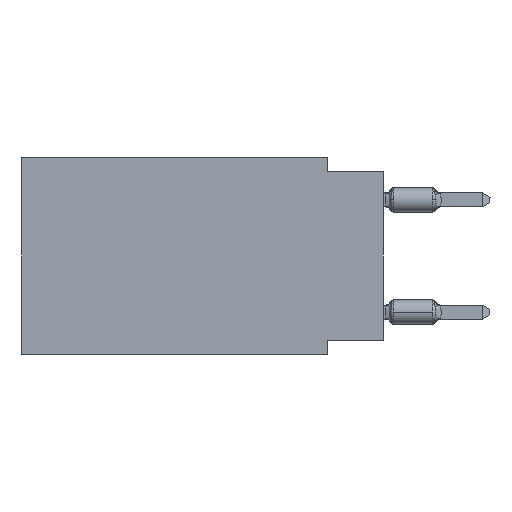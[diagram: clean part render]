
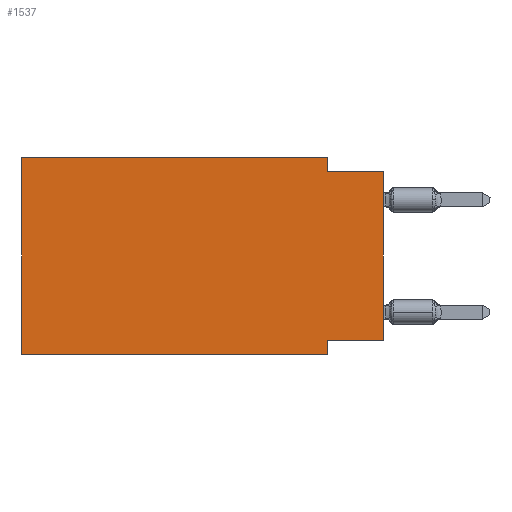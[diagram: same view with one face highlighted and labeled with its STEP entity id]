
A CAD part, left-side view. The second image highlights one B-rep face of the part: STEP entity #1537.
In plain terms, the highlighted planar face has unit normal (-1, 0, 0).
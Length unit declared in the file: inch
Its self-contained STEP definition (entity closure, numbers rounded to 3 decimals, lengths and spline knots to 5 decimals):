
#310 = VERTEX_POINT ( 'NONE', #21099 ) ;
#391 = EDGE_CURVE ( 'NONE', #17264, #3474, #10480, .T. ) ;
#471 = LINE ( 'NONE', #23432, #18059 ) ;
#589 = DIRECTION ( 'NONE',  ( 0., 0., -1. ) ) ;
#600 = VERTEX_POINT ( 'NONE', #11206 ) ;
#937 = CARTESIAN_POINT ( 'NONE',  ( 0., 0.1, -0.35 ) ) ;
#1000 = DIRECTION ( 'NONE',  ( 0., 0., 1. ) ) ;
#1537 = ADVANCED_FACE ( 'NONE', ( #15249 ), #3746, .F. ) ;
#1828 = EDGE_CURVE ( 'NONE', #600, #13780, #6998, .T. ) ;
#2610 = CARTESIAN_POINT ( 'NONE',  ( 0., 0.1, -0.35 ) ) ;
#2752 = LINE ( 'NONE', #18110, #24153 ) ;
#3033 = VECTOR ( 'NONE', #6122, 39.37008 ) ;
#3474 = VERTEX_POINT ( 'NONE', #937 ) ;
#3730 = ORIENTED_EDGE ( 'NONE', *, *, #391, .F. ) ;
#3746 = PLANE ( 'NONE',  #22382 ) ;
#3873 = DIRECTION ( 'NONE',  ( 0., 0., -1. ) ) ;
#4231 = LINE ( 'NONE', #15497, #3033 ) ;
#4282 = EDGE_CURVE ( 'NONE', #310, #13780, #10447, .T. ) ;
#5043 = DIRECTION ( 'NONE',  ( 0., -1., 0. ) ) ;
#6122 = DIRECTION ( 'NONE',  ( 0., 1., 0. ) ) ;
#6454 = CARTESIAN_POINT ( 'NONE',  ( 0., 0., -0.025 ) ) ;
#6998 = LINE ( 'NONE', #14608, #18767 ) ;
#9003 = VECTOR ( 'NONE', #19560, 39.37008 ) ;
#9133 = EDGE_CURVE ( 'NONE', #23872, #18545, #9851, .T. ) ;
#9687 = ORIENTED_EDGE ( 'NONE', *, *, #23823, .F. ) ;
#9851 = LINE ( 'NONE', #15473, #15080 ) ;
#10447 = LINE ( 'NONE', #6454, #9003 ) ;
#10480 = LINE ( 'NONE', #2610, #23742 ) ;
#11206 = CARTESIAN_POINT ( 'NONE',  ( 0., 0., -0.325 ) ) ;
#11257 = CARTESIAN_POINT ( 'NONE',  ( 0., 0.645, 0. ) ) ;
#11541 = ORIENTED_EDGE ( 'NONE', *, *, #4282, .F. ) ;
#11557 = ORIENTED_EDGE ( 'NONE', *, *, #1828, .T. ) ;
#12058 = VECTOR ( 'NONE', #5043, 39.37008 ) ;
#12615 = CARTESIAN_POINT ( 'NONE',  ( 0., 0.645, 0. ) ) ;
#12748 = EDGE_CURVE ( 'NONE', #18545, #310, #471, .T. ) ;
#13166 = CARTESIAN_POINT ( 'NONE',  ( 0., 0.1, 0. ) ) ;
#13590 = DIRECTION ( 'NONE',  ( 0., -1., 0. ) ) ;
#13748 = CARTESIAN_POINT ( 'NONE',  ( 0., 0.645, -0.35 ) ) ;
#13780 = VERTEX_POINT ( 'NONE', #19332 ) ;
#13970 = DIRECTION ( 'NONE',  ( 0., 0., -1. ) ) ;
#14608 = CARTESIAN_POINT ( 'NONE',  ( 0., 0., 0. ) ) ;
#15080 = VECTOR ( 'NONE', #13590, 39.37008 ) ;
#15249 = FACE_OUTER_BOUND ( 'NONE', #21252, .T. ) ;
#15251 = CARTESIAN_POINT ( 'NONE',  ( 0., 0.1, -0.325 ) ) ;
#15473 = CARTESIAN_POINT ( 'NONE',  ( 0., 0.645, 0. ) ) ;
#15497 = CARTESIAN_POINT ( 'NONE',  ( 0., 0., -0.325 ) ) ;
#16101 = ORIENTED_EDGE ( 'NONE', *, *, #12748, .F. ) ;
#16104 = VERTEX_POINT ( 'NONE', #13748 ) ;
#16425 = LINE ( 'NONE', #22160, #12058 ) ;
#17027 = ORIENTED_EDGE ( 'NONE', *, *, #9133, .F. ) ;
#17264 = VERTEX_POINT ( 'NONE', #15251 ) ;
#18059 = VECTOR ( 'NONE', #589, 39.37008 ) ;
#18110 = CARTESIAN_POINT ( 'NONE',  ( 0., 0.645, 0. ) ) ;
#18545 = VERTEX_POINT ( 'NONE', #13166 ) ;
#18767 = VECTOR ( 'NONE', #22234, 39.37008 ) ;
#19332 = CARTESIAN_POINT ( 'NONE',  ( 0., 0., -0.025 ) ) ;
#19499 = ORIENTED_EDGE ( 'NONE', *, *, #19780, .T. ) ;
#19560 = DIRECTION ( 'NONE',  ( 0., -1., 0. ) ) ;
#19780 = EDGE_CURVE ( 'NONE', #16104, #3474, #16425, .T. ) ;
#20566 = ORIENTED_EDGE ( 'NONE', *, *, #23633, .F. ) ;
#20982 = DIRECTION ( 'NONE',  ( 1., 0., 0. ) ) ;
#21099 = CARTESIAN_POINT ( 'NONE',  ( 0., 0.1, -0.025 ) ) ;
#21252 = EDGE_LOOP ( 'NONE', ( #11557, #11541, #16101, #17027, #9687, #19499, #3730, #20566 ) ) ;
#22160 = CARTESIAN_POINT ( 'NONE',  ( 0., 0.645, -0.35 ) ) ;
#22234 = DIRECTION ( 'NONE',  ( 0., 0., 1. ) ) ;
#22382 = AXIS2_PLACEMENT_3D ( 'NONE', #11257, #20982, #3873 ) ;
#23432 = CARTESIAN_POINT ( 'NONE',  ( 0., 0.1, 0. ) ) ;
#23633 = EDGE_CURVE ( 'NONE', #600, #17264, #4231, .T. ) ;
#23742 = VECTOR ( 'NONE', #13970, 39.37008 ) ;
#23823 = EDGE_CURVE ( 'NONE', #16104, #23872, #2752, .T. ) ;
#23872 = VERTEX_POINT ( 'NONE', #12615 ) ;
#24153 = VECTOR ( 'NONE', #1000, 39.37008 ) ;
